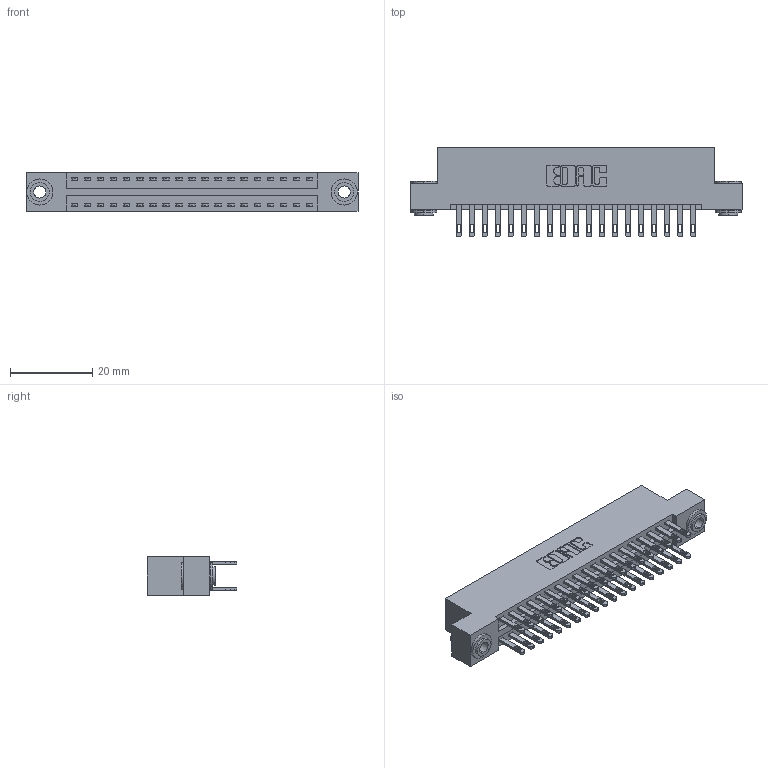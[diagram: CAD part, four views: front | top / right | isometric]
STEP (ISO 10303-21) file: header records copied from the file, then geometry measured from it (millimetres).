
FILE_DESCRIPTION (( 'STEP AP203' ), '1' );
FILE_NAME ('346-038-500-203.STEP', '2022-05-19T22:47:20', ( '' ), ( '' ), 'SwSTEP 2.0', 'SolidWorks 2020', '' );
FILE_SCHEMA (( 'CONFIG_CONTROL_DESIGN' ));
Length unit declared in the file: inch
Products named in the file (4): 345-250-002_345-250-002-102; 346-038-500-203; 345-292-001_345-293-100; 346 Part_Flush Mounting Lugs - 0.156 Dia-TH
Assembly tree (41 placements, depth 2):
  346-038-500-203
    346 Part_Flush Mounting Lugs - 0.156 Dia-TH
    345-292-001_345-293-100  x38
    345-250-002_345-250-002-102  x2
Bounding box: 80.9 x 21.84 x 9.4 mm (x, y, z)
Volume: 7827.4 mm3; surface area: 11044.3 mm2
Topology: 41 solids, 41 shells, 1998 faces, 6027 edges, 4014 vertices
Faces by surface type: plane 1202, cylinder 788, cone 8
Entity records: 16492 total; most frequent: CARTESIAN_POINT 2729, ORIENTED_EDGE 2654, DIRECTION 2489, EDGE_CURVE 1327, VECTOR 1091, LINE 1091, VERTEX_POINT 882, AXIS2_PLACEMENT_3D 699
